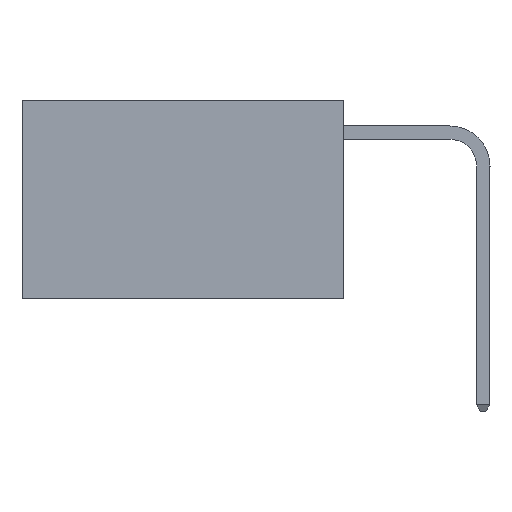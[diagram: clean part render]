
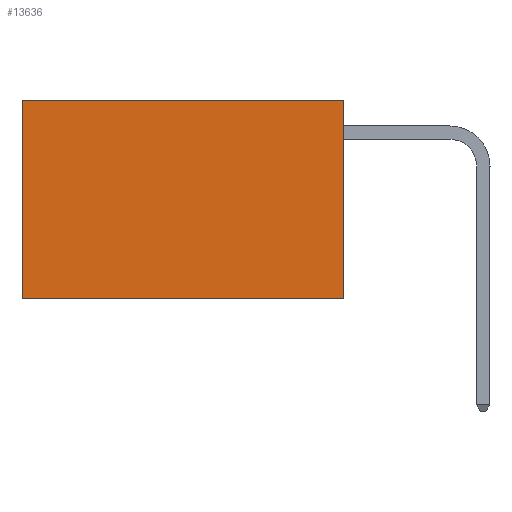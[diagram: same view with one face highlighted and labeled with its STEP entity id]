
A CAD part, left-side view. The second image highlights one B-rep face of the part: STEP entity #13636.
In plain terms, the highlighted planar face has unit normal (-1, 0, 0).
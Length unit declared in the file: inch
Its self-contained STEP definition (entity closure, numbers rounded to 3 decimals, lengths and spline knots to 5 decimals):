
#435 = VERTEX_POINT ( 'NONE', #5150 ) ;
#982 = EDGE_CURVE ( 'NONE', #13092, #4685, #2573, .T. ) ;
#1218 = DIRECTION ( 'NONE',  ( 0., 0., -1. ) ) ;
#1285 = VECTOR ( 'NONE', #6063, 39.37008 ) ;
#1642 = EDGE_CURVE ( 'NONE', #435, #8411, #8270, .T. ) ;
#1918 = VECTOR ( 'NONE', #3655, 39.37008 ) ;
#2230 = DIRECTION ( 'NONE',  ( 0., 0., -1. ) ) ;
#2328 = ORIENTED_EDGE ( 'NONE', *, *, #5863, .F. ) ;
#2573 = LINE ( 'NONE', #8836, #5162 ) ;
#3263 = CARTESIAN_POINT ( 'NONE',  ( 0.2625, 0., 0. ) ) ;
#3655 = DIRECTION ( 'NONE',  ( 0., 0., -1. ) ) ;
#4685 = VERTEX_POINT ( 'NONE', #12505 ) ;
#5150 = CARTESIAN_POINT ( 'NONE',  ( 0.2625, 0., 0. ) ) ;
#5162 = VECTOR ( 'NONE', #2230, 39.37008 ) ;
#5863 = EDGE_CURVE ( 'NONE', #8411, #4685, #10865, .T. ) ;
#6050 = ORIENTED_EDGE ( 'NONE', *, *, #1642, .F. ) ;
#6063 = DIRECTION ( 'NONE',  ( 0., 1., 0. ) ) ;
#6210 = PLANE ( 'NONE',  #13302 ) ;
#6308 = EDGE_LOOP ( 'NONE', ( #8277, #2328, #6050, #8935 ) ) ;
#6747 = EDGE_CURVE ( 'NONE', #435, #13092, #6913, .T. ) ;
#6827 = FACE_OUTER_BOUND ( 'NONE', #6308, .T. ) ;
#6913 = LINE ( 'NONE', #3263, #14460 ) ;
#7351 = CARTESIAN_POINT ( 'NONE',  ( 0.2625, 0., 0. ) ) ;
#8029 = CARTESIAN_POINT ( 'NONE',  ( 0.2625, 0.6, 0. ) ) ;
#8270 = LINE ( 'NONE', #8318, #1918 ) ;
#8277 = ORIENTED_EDGE ( 'NONE', *, *, #982, .T. ) ;
#8318 = CARTESIAN_POINT ( 'NONE',  ( 0.2625, 0., 0. ) ) ;
#8395 = DIRECTION ( 'NONE',  ( 1., 0., 0. ) ) ;
#8411 = VERTEX_POINT ( 'NONE', #8492 ) ;
#8492 = CARTESIAN_POINT ( 'NONE',  ( 0.2625, 0., -0.37 ) ) ;
#8836 = CARTESIAN_POINT ( 'NONE',  ( 0.2625, 0.6, 0. ) ) ;
#8935 = ORIENTED_EDGE ( 'NONE', *, *, #6747, .T. ) ;
#10865 = LINE ( 'NONE', #13349, #1285 ) ;
#12505 = CARTESIAN_POINT ( 'NONE',  ( 0.2625, 0.6, -0.37 ) ) ;
#13092 = VERTEX_POINT ( 'NONE', #8029 ) ;
#13302 = AXIS2_PLACEMENT_3D ( 'NONE', #7351, #8395, #1218 ) ;
#13349 = CARTESIAN_POINT ( 'NONE',  ( 0.2625, 0., -0.37 ) ) ;
#13636 = ADVANCED_FACE ( 'NONE', ( #6827 ), #6210, .F. ) ;
#14096 = DIRECTION ( 'NONE',  ( 0., 1., 0. ) ) ;
#14460 = VECTOR ( 'NONE', #14096, 39.37008 ) ;
